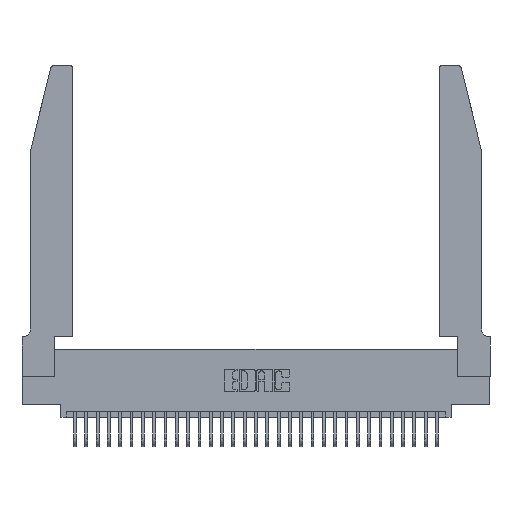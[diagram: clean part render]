
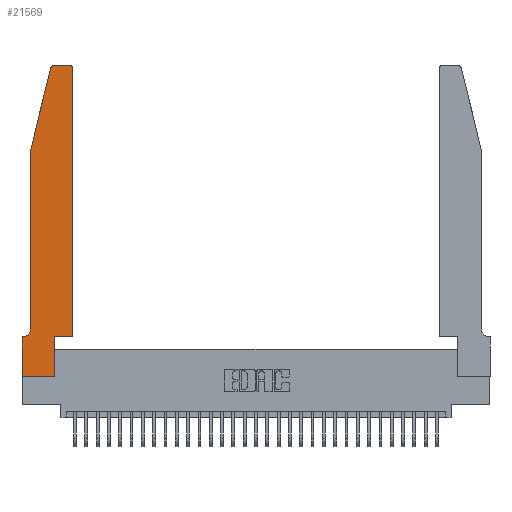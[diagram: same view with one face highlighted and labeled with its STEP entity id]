
A CAD part, top view. The second image highlights one B-rep face of the part: STEP entity #21569.
In plain terms, the highlighted planar face has unit normal (0, 0, 1).
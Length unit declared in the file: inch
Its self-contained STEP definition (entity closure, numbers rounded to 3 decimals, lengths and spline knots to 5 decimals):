
#599 = VERTEX_POINT ( 'NONE', #4844 ) ;
#811 = DIRECTION ( 'NONE',  ( 1., 0., 0. ) ) ;
#914 = DIRECTION ( 'NONE',  ( 0., -1., 0. ) ) ;
#1035 = ORIENTED_EDGE ( 'NONE', *, *, #21719, .T. ) ;
#2076 = EDGE_CURVE ( 'NONE', #12449, #31645, #20446, .T. ) ;
#3054 = FACE_OUTER_BOUND ( 'NONE', #26456, .T. ) ;
#3178 = ORIENTED_EDGE ( 'NONE', *, *, #2076, .T. ) ;
#4844 = CARTESIAN_POINT ( 'NONE',  ( 0.0055, 0.35, 0.37 ) ) ;
#5020 = AXIS2_PLACEMENT_3D ( 'NONE', #31958, #16704, #811 ) ;
#5357 = ORIENTED_EDGE ( 'NONE', *, *, #27381, .T. ) ;
#5782 = EDGE_CURVE ( 'NONE', #599, #19202, #27824, .T. ) ;
#5815 = CARTESIAN_POINT ( 'NONE',  ( 0.4505, 0.35, 0.37 ) ) ;
#6204 = AXIS2_PLACEMENT_3D ( 'NONE', #9535, #12223, #30085 ) ;
#6787 = VERTEX_POINT ( 'NONE', #10229 ) ;
#7257 = CARTESIAN_POINT ( 'NONE',  ( 0., 0., 0.37 ) ) ;
#7448 = DIRECTION ( 'NONE',  ( 0., -1., 0. ) ) ;
#7706 = VECTOR ( 'NONE', #18167, 39.37008 ) ;
#7767 = VERTEX_POINT ( 'NONE', #26913 ) ;
#7967 = EDGE_CURVE ( 'NONE', #21431, #14431, #16807, .T. ) ;
#8183 = VECTOR ( 'NONE', #30440, 39.37008 ) ;
#8293 = DIRECTION ( 'NONE',  ( -0.239, -0.971, 0. ) ) ;
#8534 = VECTOR ( 'NONE', #29329, 39.37008 ) ;
#8635 = CARTESIAN_POINT ( 'NONE',  ( 0.284, 2.72, 0.37 ) ) ;
#8737 = EDGE_CURVE ( 'NONE', #31645, #9150, #13140, .T. ) ;
#9057 = CARTESIAN_POINT ( 'NONE',  ( 0.4505, 2.72, 0.37 ) ) ;
#9150 = VERTEX_POINT ( 'NONE', #13545 ) ;
#9193 = EDGE_CURVE ( 'NONE', #6787, #21431, #14722, .T. ) ;
#9258 = AXIS2_PLACEMENT_3D ( 'NONE', #8635, #26705, #11342 ) ;
#9535 = CARTESIAN_POINT ( 'NONE',  ( 0., 0.35, 0.37 ) ) ;
#9877 = VERTEX_POINT ( 'NONE', #10983 ) ;
#9909 = CARTESIAN_POINT ( 'NONE',  ( 0.4505, 0.35, 0.37 ) ) ;
#10229 = CARTESIAN_POINT ( 'NONE',  ( 0.2865, 0.35, 0.37 ) ) ;
#10983 = CARTESIAN_POINT ( 'NONE',  ( 0.284, 2.75, 0.37 ) ) ;
#10988 = CARTESIAN_POINT ( 'NONE',  ( 0.0055, 0.42, 0.37 ) ) ;
#11026 = DIRECTION ( 'NONE',  ( 1., 0., 0. ) ) ;
#11041 = VERTEX_POINT ( 'NONE', #17831 ) ;
#11342 = DIRECTION ( 'NONE',  ( 1., 0., 0. ) ) ;
#11408 = CARTESIAN_POINT ( 'NONE',  ( 0.0755, 2., 0.37 ) ) ;
#11485 = VECTOR ( 'NONE', #28893, 39.37008 ) ;
#12223 = DIRECTION ( 'NONE',  ( 0., 0., 1. ) ) ;
#12449 = VERTEX_POINT ( 'NONE', #13925 ) ;
#13140 = LINE ( 'NONE', #19408, #19182 ) ;
#13545 = CARTESIAN_POINT ( 'NONE',  ( 0.0755, 0.42, 0.37 ) ) ;
#13630 = DIRECTION ( 'NONE',  ( -1., 0., 0. ) ) ;
#13731 = CARTESIAN_POINT ( 'NONE',  ( 0.0755, 0.35, 0.37 ) ) ;
#13925 = CARTESIAN_POINT ( 'NONE',  ( 0.25487, 2.72718, 0.37 ) ) ;
#14431 = VERTEX_POINT ( 'NONE', #9057 ) ;
#14722 = LINE ( 'NONE', #5815, #27511 ) ;
#14926 = VECTOR ( 'NONE', #30465, 39.37008 ) ;
#15003 = EDGE_CURVE ( 'NONE', #24000, #9877, #16340, .T. ) ;
#15567 = CARTESIAN_POINT ( 'NONE',  ( 0.2865, 0.35, 0.37 ) ) ;
#16145 = CARTESIAN_POINT ( 'NONE',  ( 0.0755, 2., 0.37 ) ) ;
#16340 = LINE ( 'NONE', #29107, #8534 ) ;
#16596 = CIRCLE ( 'NONE', #31503, 0.07 ) ;
#16704 = DIRECTION ( 'NONE',  ( 0., 0., 1. ) ) ;
#16807 = LINE ( 'NONE', #9909, #8183 ) ;
#16812 = ORIENTED_EDGE ( 'NONE', *, *, #27725, .T. ) ;
#17831 = CARTESIAN_POINT ( 'NONE',  ( 0., 0., 0.37 ) ) ;
#18167 = DIRECTION ( 'NONE',  ( 0., 1., 0. ) ) ;
#19109 = VECTOR ( 'NONE', #7448, 39.37008 ) ;
#19182 = VECTOR ( 'NONE', #914, 39.37008 ) ;
#19194 = CIRCLE ( 'NONE', #5020, 0.03 ) ;
#19202 = VERTEX_POINT ( 'NONE', #26207 ) ;
#19408 = CARTESIAN_POINT ( 'NONE',  ( 0.0755, 2., 0.37 ) ) ;
#20446 = LINE ( 'NONE', #16145, #26402 ) ;
#21073 = CIRCLE ( 'NONE', #9258, 0.03 ) ;
#21214 = ORIENTED_EDGE ( 'NONE', *, *, #5782, .T. ) ;
#21431 = VERTEX_POINT ( 'NONE', #24457 ) ;
#21569 = ADVANCED_FACE ( 'NONE', ( #3054 ), #27555, .T. ) ;
#21719 = EDGE_CURVE ( 'NONE', #19202, #11041, #25092, .T. ) ;
#22005 = ORIENTED_EDGE ( 'NONE', *, *, #24162, .T. ) ;
#22403 = ORIENTED_EDGE ( 'NONE', *, *, #15003, .T. ) ;
#24000 = VERTEX_POINT ( 'NONE', #27052 ) ;
#24162 = EDGE_CURVE ( 'NONE', #11041, #7767, #28484, .T. ) ;
#24420 = ORIENTED_EDGE ( 'NONE', *, *, #7967, .T. ) ;
#24457 = CARTESIAN_POINT ( 'NONE',  ( 0.4505, 0.35, 0.37 ) ) ;
#25092 = LINE ( 'NONE', #25580, #19109 ) ;
#25580 = CARTESIAN_POINT ( 'NONE',  ( 0., 0., 0.37 ) ) ;
#26207 = CARTESIAN_POINT ( 'NONE',  ( 0., 0.35, 0.37 ) ) ;
#26393 = ORIENTED_EDGE ( 'NONE', *, *, #32902, .T. ) ;
#26402 = VECTOR ( 'NONE', #8293, 39.37008 ) ;
#26456 = EDGE_LOOP ( 'NONE', ( #22403, #29932, #3178, #32319, #26393, #21214, #1035, #22005, #16812, #30354, #24420, #5357 ) ) ;
#26705 = DIRECTION ( 'NONE',  ( 0., 0., 1. ) ) ;
#26913 = CARTESIAN_POINT ( 'NONE',  ( 0.2865, 0., 0.37 ) ) ;
#27052 = CARTESIAN_POINT ( 'NONE',  ( 0.4205, 2.75, 0.37 ) ) ;
#27381 = EDGE_CURVE ( 'NONE', #14431, #24000, #19194, .T. ) ;
#27511 = VECTOR ( 'NONE', #11026, 39.37008 ) ;
#27555 = PLANE ( 'NONE',  #6204 ) ;
#27725 = EDGE_CURVE ( 'NONE', #7767, #6787, #28323, .T. ) ;
#27824 = LINE ( 'NONE', #13731, #11485 ) ;
#28323 = LINE ( 'NONE', #15567, #7706 ) ;
#28484 = LINE ( 'NONE', #7257, #14926 ) ;
#28862 = EDGE_CURVE ( 'NONE', #9877, #12449, #21073, .T. ) ;
#28893 = DIRECTION ( 'NONE',  ( -1., 0., 0. ) ) ;
#28894 = DIRECTION ( 'NONE',  ( 0., 0., -1. ) ) ;
#29107 = CARTESIAN_POINT ( 'NONE',  ( 0.2605, 2.75, 0.37 ) ) ;
#29329 = DIRECTION ( 'NONE',  ( -1., 0., 0. ) ) ;
#29932 = ORIENTED_EDGE ( 'NONE', *, *, #28862, .T. ) ;
#30085 = DIRECTION ( 'NONE',  ( 1., 0., 0. ) ) ;
#30354 = ORIENTED_EDGE ( 'NONE', *, *, #9193, .T. ) ;
#30440 = DIRECTION ( 'NONE',  ( 0., 1., 0. ) ) ;
#30465 = DIRECTION ( 'NONE',  ( 1., 0., 0. ) ) ;
#31503 = AXIS2_PLACEMENT_3D ( 'NONE', #10988, #28894, #13630 ) ;
#31645 = VERTEX_POINT ( 'NONE', #11408 ) ;
#31958 = CARTESIAN_POINT ( 'NONE',  ( 0.4205, 2.72, 0.37 ) ) ;
#32319 = ORIENTED_EDGE ( 'NONE', *, *, #8737, .T. ) ;
#32902 = EDGE_CURVE ( 'NONE', #9150, #599, #16596, .T. ) ;
